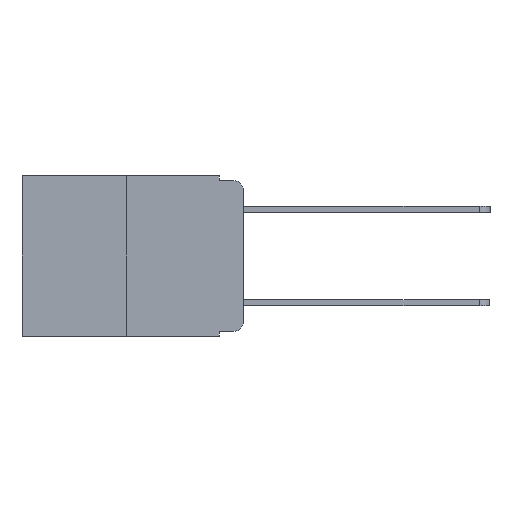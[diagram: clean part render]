
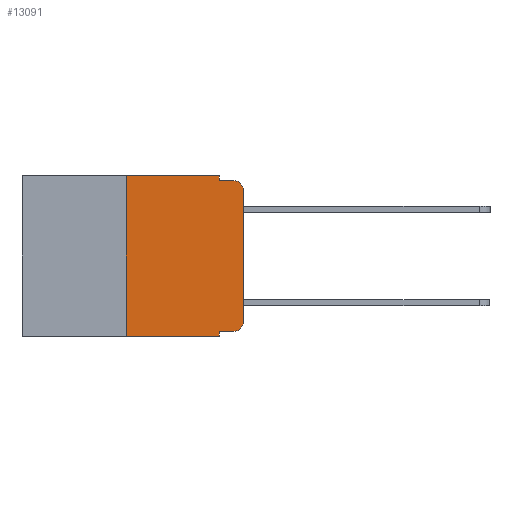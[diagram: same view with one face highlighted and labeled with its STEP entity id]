
A CAD part, left-side view. The second image highlights one B-rep face of the part: STEP entity #13091.
In plain terms, the highlighted planar face has unit normal (-1, 0, 0).
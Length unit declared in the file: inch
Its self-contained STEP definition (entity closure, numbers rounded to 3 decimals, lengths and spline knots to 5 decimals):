
#100 = ORIENTED_EDGE ( 'NONE', *, *, #1252, .F. ) ;
#382 = DIRECTION ( 'NONE',  ( 0., 0., 1. ) ) ;
#653 = LINE ( 'NONE', #2818, #21007 ) ;
#1252 = EDGE_CURVE ( 'NONE', #13744, #15560, #653, .T. ) ;
#1504 = DIRECTION ( 'NONE',  ( 0., 0., -1. ) ) ;
#2119 = CARTESIAN_POINT ( 'NONE',  ( 0., 0.051, -0.01 ) ) ;
#2247 = CARTESIAN_POINT ( 'NONE',  ( 0., 0.25, 0. ) ) ;
#2794 = CARTESIAN_POINT ( 'NONE',  ( 0., 0.02, -0.01 ) ) ;
#2818 = CARTESIAN_POINT ( 'NONE',  ( 0., 0.25, 0. ) ) ;
#3080 = CARTESIAN_POINT ( 'NONE',  ( 0., 0.473, -0.343 ) ) ;
#3152 = CARTESIAN_POINT ( 'NONE',  ( 0., 0.02, -0.03 ) ) ;
#3473 = CARTESIAN_POINT ( 'NONE',  ( 0., 0.051, -0.01 ) ) ;
#4177 = LINE ( 'NONE', #24045, #24268 ) ;
#4666 = DIRECTION ( 'NONE',  ( 0., -1., 0. ) ) ;
#5101 = DIRECTION ( 'NONE',  ( 0., -1., 0. ) ) ;
#5186 = DIRECTION ( 'NONE',  ( 0., 0., -1. ) ) ;
#5217 = ORIENTED_EDGE ( 'NONE', *, *, #8017, .F. ) ;
#6619 = CARTESIAN_POINT ( 'NONE',  ( 0., 0.051, -0.333 ) ) ;
#6720 = FACE_OUTER_BOUND ( 'NONE', #24704, .T. ) ;
#6982 = VERTEX_POINT ( 'NONE', #2119 ) ;
#7035 = PLANE ( 'NONE',  #11971 ) ;
#8017 = EDGE_CURVE ( 'NONE', #11279, #6982, #24558, .T. ) ;
#8128 = VERTEX_POINT ( 'NONE', #25257 ) ;
#8983 = DIRECTION ( 'NONE',  ( 1., 0., 0. ) ) ;
#10381 = VERTEX_POINT ( 'NONE', #6619 ) ;
#10696 = LINE ( 'NONE', #3080, #20431 ) ;
#11279 = VERTEX_POINT ( 'NONE', #24924 ) ;
#11295 = DIRECTION ( 'NONE',  ( -1., 0., 0. ) ) ;
#11944 = EDGE_CURVE ( 'NONE', #6982, #18362, #22587, .T. ) ;
#11971 = AXIS2_PLACEMENT_3D ( 'NONE', #18684, #8983, #22577 ) ;
#12443 = CIRCLE ( 'NONE', #19705, 0.02 ) ;
#12631 = ORIENTED_EDGE ( 'NONE', *, *, #15044, .T. ) ;
#12967 = VECTOR ( 'NONE', #15388, 39.37008 ) ;
#13051 = CIRCLE ( 'NONE', #13325, 0.02 ) ;
#13091 = ADVANCED_FACE ( 'NONE', ( #6720 ), #7035, .F. ) ;
#13325 = AXIS2_PLACEMENT_3D ( 'NONE', #22908, #11295, #24788 ) ;
#13541 = CARTESIAN_POINT ( 'NONE',  ( 0., 0., -0.313 ) ) ;
#13623 = EDGE_CURVE ( 'NONE', #15560, #11279, #4177, .T. ) ;
#13744 = VERTEX_POINT ( 'NONE', #21023 ) ;
#14513 = VERTEX_POINT ( 'NONE', #13541 ) ;
#14691 = ORIENTED_EDGE ( 'NONE', *, *, #18455, .T. ) ;
#14938 = CARTESIAN_POINT ( 'NONE',  ( 0., 0., -0.03 ) ) ;
#14988 = VECTOR ( 'NONE', #18159, 39.37008 ) ;
#15044 = EDGE_CURVE ( 'NONE', #16010, #14513, #13051, .T. ) ;
#15361 = CARTESIAN_POINT ( 'NONE',  ( 0., 0.051, 0. ) ) ;
#15388 = DIRECTION ( 'NONE',  ( 0., -1., 0. ) ) ;
#15560 = VERTEX_POINT ( 'NONE', #2247 ) ;
#16010 = VERTEX_POINT ( 'NONE', #19571 ) ;
#16163 = CARTESIAN_POINT ( 'NONE',  ( 0., 0., 0. ) ) ;
#16895 = DIRECTION ( 'NONE',  ( -1., 0., 0. ) ) ;
#16942 = DIRECTION ( 'NONE',  ( 0., 0., -1. ) ) ;
#17233 = VECTOR ( 'NONE', #16942, 39.37008 ) ;
#18159 = DIRECTION ( 'NONE',  ( 0., 0., 1. ) ) ;
#18362 = VERTEX_POINT ( 'NONE', #2794 ) ;
#18455 = EDGE_CURVE ( 'NONE', #18476, #18362, #12443, .T. ) ;
#18476 = VERTEX_POINT ( 'NONE', #14938 ) ;
#18654 = ORIENTED_EDGE ( 'NONE', *, *, #13623, .F. ) ;
#18684 = CARTESIAN_POINT ( 'NONE',  ( 0., 0.473, 0. ) ) ;
#19098 = CARTESIAN_POINT ( 'NONE',  ( 0., 0.051, -0.333 ) ) ;
#19463 = VECTOR ( 'NONE', #1504, 39.37008 ) ;
#19571 = CARTESIAN_POINT ( 'NONE',  ( 0., 0.02, -0.333 ) ) ;
#19705 = AXIS2_PLACEMENT_3D ( 'NONE', #3152, #16895, #5186 ) ;
#20138 = LINE ( 'NONE', #16163, #14988 ) ;
#20240 = EDGE_CURVE ( 'NONE', #10381, #16010, #22668, .T. ) ;
#20431 = VECTOR ( 'NONE', #5101, 39.37008 ) ;
#21007 = VECTOR ( 'NONE', #382, 39.37008 ) ;
#21023 = CARTESIAN_POINT ( 'NONE',  ( 0., 0.25, -0.343 ) ) ;
#21365 = VECTOR ( 'NONE', #23011, 39.37008 ) ;
#22348 = EDGE_CURVE ( 'NONE', #14513, #18476, #20138, .T. ) ;
#22528 = EDGE_CURVE ( 'NONE', #13744, #8128, #10696, .T. ) ;
#22557 = ORIENTED_EDGE ( 'NONE', *, *, #22348, .T. ) ;
#22577 = DIRECTION ( 'NONE',  ( 0., 0., -1. ) ) ;
#22587 = LINE ( 'NONE', #3473, #21365 ) ;
#22626 = ORIENTED_EDGE ( 'NONE', *, *, #25344, .F. ) ;
#22668 = LINE ( 'NONE', #19098, #12967 ) ;
#22681 = CARTESIAN_POINT ( 'NONE',  ( 0., 0.051, 0. ) ) ;
#22863 = ORIENTED_EDGE ( 'NONE', *, *, #11944, .F. ) ;
#22908 = CARTESIAN_POINT ( 'NONE',  ( 0., 0.02, -0.313 ) ) ;
#23011 = DIRECTION ( 'NONE',  ( 0., -1., 0. ) ) ;
#23509 = ORIENTED_EDGE ( 'NONE', *, *, #22528, .T. ) ;
#23811 = ORIENTED_EDGE ( 'NONE', *, *, #20240, .T. ) ;
#24045 = CARTESIAN_POINT ( 'NONE',  ( 0., 0.473, 0. ) ) ;
#24165 = LINE ( 'NONE', #22681, #17233 ) ;
#24268 = VECTOR ( 'NONE', #4666, 39.37008 ) ;
#24558 = LINE ( 'NONE', #15361, #19463 ) ;
#24704 = EDGE_LOOP ( 'NONE', ( #22557, #14691, #22863, #5217, #18654, #100, #23509, #22626, #23811, #12631 ) ) ;
#24788 = DIRECTION ( 'NONE',  ( 0., 0., -1. ) ) ;
#24924 = CARTESIAN_POINT ( 'NONE',  ( 0., 0.051, 0. ) ) ;
#25257 = CARTESIAN_POINT ( 'NONE',  ( 0., 0.051, -0.343 ) ) ;
#25344 = EDGE_CURVE ( 'NONE', #10381, #8128, #24165, .T. ) ;
